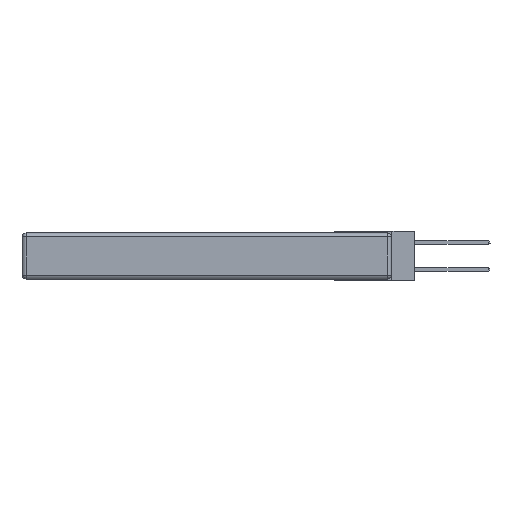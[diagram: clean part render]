
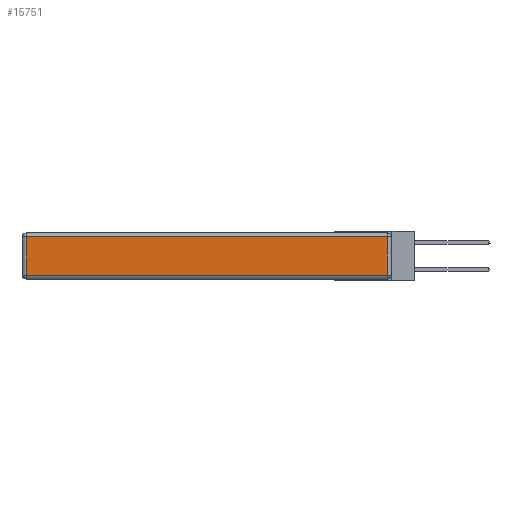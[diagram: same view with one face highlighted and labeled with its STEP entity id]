
A CAD part, left-side view. The second image highlights one B-rep face of the part: STEP entity #15751.
In plain terms, the highlighted planar face has unit normal (-1, 0, 0).
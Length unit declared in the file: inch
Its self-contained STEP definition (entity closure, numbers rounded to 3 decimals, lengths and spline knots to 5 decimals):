
#115 = VECTOR ( 'NONE', #9642, 39.37008 ) ;
#859 = CARTESIAN_POINT ( 'NONE',  ( 0., 2.72, -0.343 ) ) ;
#1329 = VECTOR ( 'NONE', #10632, 39.37008 ) ;
#1693 = PLANE ( 'NONE',  #16148 ) ;
#2016 = ORIENTED_EDGE ( 'NONE', *, *, #6549, .T. ) ;
#2444 = FACE_OUTER_BOUND ( 'NONE', #3331, .T. ) ;
#2758 = EDGE_CURVE ( 'NONE', #6359, #7588, #5082, .T. ) ;
#3331 = EDGE_LOOP ( 'NONE', ( #14536, #6793, #16080, #2016 ) ) ;
#3555 = LINE ( 'NONE', #859, #115 ) ;
#4407 = DIRECTION ( 'NONE',  ( 0., 1., 0. ) ) ;
#5082 = LINE ( 'NONE', #5370, #13362 ) ;
#5370 = CARTESIAN_POINT ( 'NONE',  ( 0., 0.03, -0.343 ) ) ;
#5559 = CARTESIAN_POINT ( 'NONE',  ( 0., 0., -0.343 ) ) ;
#6169 = CARTESIAN_POINT ( 'NONE',  ( 0., 2.72, -0.03 ) ) ;
#6359 = VERTEX_POINT ( 'NONE', #7316 ) ;
#6549 = EDGE_CURVE ( 'NONE', #7556, #16102, #3555, .T. ) ;
#6793 = ORIENTED_EDGE ( 'NONE', *, *, #2758, .T. ) ;
#6878 = DIRECTION ( 'NONE',  ( 0., 0., 1. ) ) ;
#7316 = CARTESIAN_POINT ( 'NONE',  ( 0., 0.03, -0.313 ) ) ;
#7556 = VERTEX_POINT ( 'NONE', #6169 ) ;
#7588 = VERTEX_POINT ( 'NONE', #13210 ) ;
#8629 = EDGE_CURVE ( 'NONE', #7588, #7556, #8673, .T. ) ;
#8673 = LINE ( 'NONE', #12085, #13768 ) ;
#9642 = DIRECTION ( 'NONE',  ( 0., 0., -1. ) ) ;
#10632 = DIRECTION ( 'NONE',  ( 0., -1., 0. ) ) ;
#10692 = DIRECTION ( 'NONE',  ( -1., 0., 0. ) ) ;
#10794 = CARTESIAN_POINT ( 'NONE',  ( 0., 0., -0.313 ) ) ;
#11023 = EDGE_CURVE ( 'NONE', #16102, #6359, #11434, .T. ) ;
#11434 = LINE ( 'NONE', #10794, #1329 ) ;
#12085 = CARTESIAN_POINT ( 'NONE',  ( 0., 2.75, -0.03 ) ) ;
#13210 = CARTESIAN_POINT ( 'NONE',  ( 0., 0.03, -0.03 ) ) ;
#13335 = DIRECTION ( 'NONE',  ( 0., 0., 1. ) ) ;
#13362 = VECTOR ( 'NONE', #6878, 39.37008 ) ;
#13768 = VECTOR ( 'NONE', #4407, 39.37008 ) ;
#14536 = ORIENTED_EDGE ( 'NONE', *, *, #11023, .T. ) ;
#14551 = CARTESIAN_POINT ( 'NONE',  ( 0., 2.72, -0.313 ) ) ;
#15751 = ADVANCED_FACE ( 'NONE', ( #2444 ), #1693, .T. ) ;
#16080 = ORIENTED_EDGE ( 'NONE', *, *, #8629, .T. ) ;
#16102 = VERTEX_POINT ( 'NONE', #14551 ) ;
#16148 = AXIS2_PLACEMENT_3D ( 'NONE', #5559, #10692, #13335 ) ;
